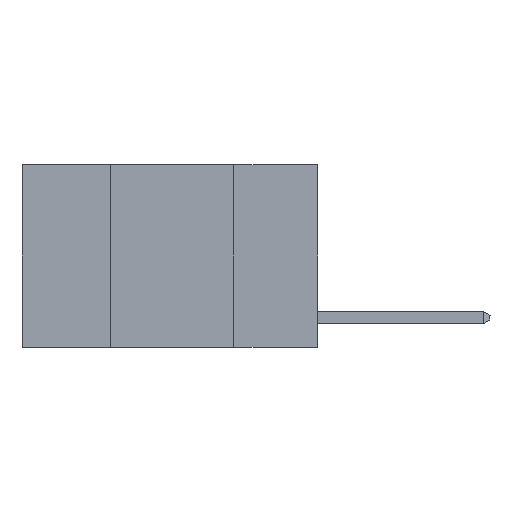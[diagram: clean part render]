
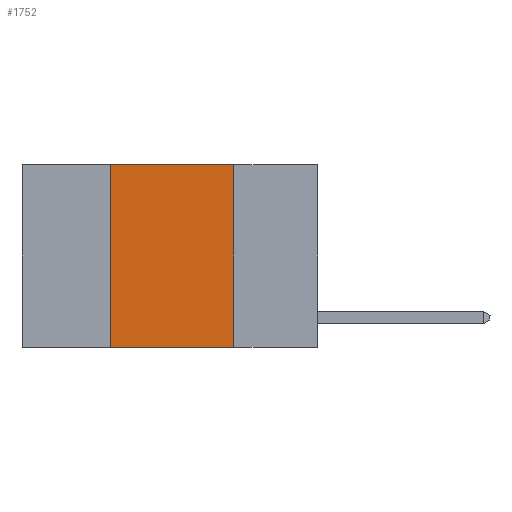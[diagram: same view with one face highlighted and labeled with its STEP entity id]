
A CAD part, left-side view. The second image highlights one B-rep face of the part: STEP entity #1752.
In plain terms, the highlighted planar face has unit normal (-1, 0, 0).
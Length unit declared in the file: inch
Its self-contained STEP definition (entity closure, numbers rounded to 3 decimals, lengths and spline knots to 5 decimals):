
#6 = DIRECTION ( 'NONE',  ( 0., 0., -1. ) ) ;
#99 = CARTESIAN_POINT ( 'NONE',  ( 0., 0.6, 0. ) ) ;
#699 = PLANE ( 'NONE',  #5285 ) ;
#1115 = LINE ( 'NONE', #10148, #5840 ) ;
#1372 = VECTOR ( 'NONE', #19067, 39.37008 ) ;
#1491 = EDGE_CURVE ( 'NONE', #7206, #5787, #1115, .T. ) ;
#1704 = LINE ( 'NONE', #14855, #19180 ) ;
#1752 = ADVANCED_FACE ( 'NONE', ( #28984 ), #699, .F. ) ;
#2226 = VERTEX_POINT ( 'NONE', #28185 ) ;
#2256 = VECTOR ( 'NONE', #20798, 39.37008 ) ;
#5285 = AXIS2_PLACEMENT_3D ( 'NONE', #99, #29528, #6 ) ;
#5461 = CARTESIAN_POINT ( 'NONE',  ( 0., 0.6, 0. ) ) ;
#5787 = VERTEX_POINT ( 'NONE', #8078 ) ;
#5840 = VECTOR ( 'NONE', #26847, 39.37008 ) ;
#7206 = VERTEX_POINT ( 'NONE', #15432 ) ;
#7730 = ORIENTED_EDGE ( 'NONE', *, *, #9885, .F. ) ;
#8078 = CARTESIAN_POINT ( 'NONE',  ( 0., 0.42, 0. ) ) ;
#9885 = EDGE_CURVE ( 'NONE', #27736, #2226, #20466, .T. ) ;
#10148 = CARTESIAN_POINT ( 'NONE',  ( 0., 0.42, 0. ) ) ;
#13029 = ORIENTED_EDGE ( 'NONE', *, *, #26155, .F. ) ;
#13616 = EDGE_CURVE ( 'NONE', #7206, #2226, #1704, .T. ) ;
#14855 = CARTESIAN_POINT ( 'NONE',  ( 0., 0.6, -0.37 ) ) ;
#15432 = CARTESIAN_POINT ( 'NONE',  ( 0., 0.42, -0.37 ) ) ;
#15521 = CARTESIAN_POINT ( 'NONE',  ( 0., 0.17, 0. ) ) ;
#16210 = ORIENTED_EDGE ( 'NONE', *, *, #13616, .T. ) ;
#16235 = CARTESIAN_POINT ( 'NONE',  ( 0., 0.17, 0. ) ) ;
#17164 = DIRECTION ( 'NONE',  ( 0., -1., 0. ) ) ;
#18026 = EDGE_LOOP ( 'NONE', ( #7730, #13029, #23707, #16210 ) ) ;
#19067 = DIRECTION ( 'NONE',  ( 0., -1., 0. ) ) ;
#19180 = VECTOR ( 'NONE', #17164, 39.37008 ) ;
#20466 = LINE ( 'NONE', #16235, #2256 ) ;
#20798 = DIRECTION ( 'NONE',  ( 0., 0., -1. ) ) ;
#23707 = ORIENTED_EDGE ( 'NONE', *, *, #1491, .F. ) ;
#24937 = LINE ( 'NONE', #5461, #1372 ) ;
#26155 = EDGE_CURVE ( 'NONE', #5787, #27736, #24937, .T. ) ;
#26847 = DIRECTION ( 'NONE',  ( 0., 0., 1. ) ) ;
#27736 = VERTEX_POINT ( 'NONE', #15521 ) ;
#28185 = CARTESIAN_POINT ( 'NONE',  ( 0., 0.17, -0.37 ) ) ;
#28984 = FACE_OUTER_BOUND ( 'NONE', #18026, .T. ) ;
#29528 = DIRECTION ( 'NONE',  ( 1., 0., 0. ) ) ;
